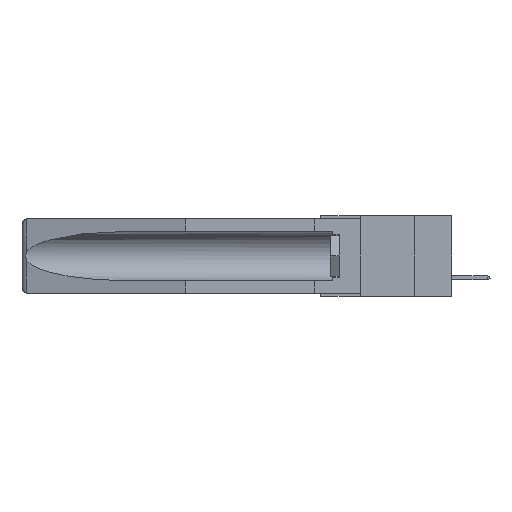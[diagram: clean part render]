
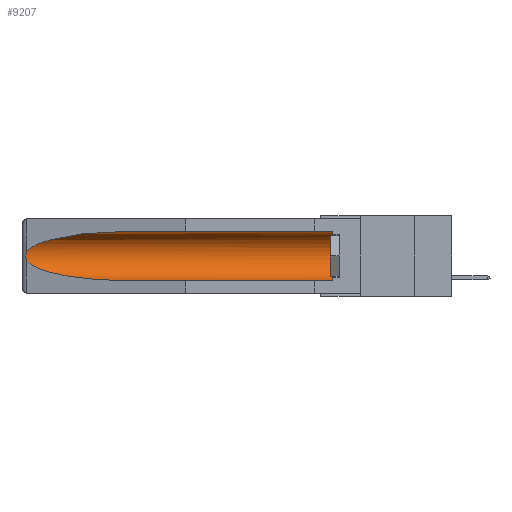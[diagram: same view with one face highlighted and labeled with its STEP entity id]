
A CAD part, left-side view. The second image highlights one B-rep face of the part: STEP entity #9207.
In plain terms, the highlighted cylindrical face has radius 2.857 mm (diameter 5.715 mm), a partial arc.
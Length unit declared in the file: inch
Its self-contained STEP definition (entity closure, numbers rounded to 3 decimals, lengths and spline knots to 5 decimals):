
#375 = B_SPLINE_CURVE_WITH_KNOTS ( 'NONE', 3,
 ( #19235, #2201, #18128, #20437, #11362, #25217, #8848, #13440, #29422, #16151 ),
 .UNSPECIFIED., .F., .F.,
 ( 4, 2, 2, 2, 4 ),
 ( 0., 0.00029, 0.00058, 0.00087, 0.00117 ),
 .UNSPECIFIED. ) ;
#1350 = ORIENTED_EDGE ( 'NONE', *, *, #18300, .T. ) ;
#1431 = VERTEX_POINT ( 'NONE', #3185 ) ;
#2054 = EDGE_CURVE ( 'NONE', #2586, #7337, #375, .T. ) ;
#2201 = CARTESIAN_POINT ( 'NONE',  ( 0.26597, 1.52961, -0.15275 ) ) ;
#2586 = VERTEX_POINT ( 'NONE', #4891 ) ;
#2819 = CARTESIAN_POINT ( 'NONE',  ( 0.155, 1.07973, -0.284 ) ) ;
#3185 = CARTESIAN_POINT ( 'NONE',  ( 0.155, 1.07973, -0.059 ) ) ;
#4318 = CARTESIAN_POINT ( 'NONE',  ( 0.155, 0.126, -0.059 ) ) ;
#4891 = CARTESIAN_POINT ( 'NONE',  ( 0.26537, 1.52718, -0.14972 ) ) ;
#6897 = CARTESIAN_POINT ( 'NONE',  ( 0.155, 0.126, -0.284 ) ) ;
#6979 =( BOUNDED_CURVE ( )  B_SPLINE_CURVE ( 3, ( #18238, #9272, #11580, #7093 ),
 .UNSPECIFIED., .F., .F. ) 
 B_SPLINE_CURVE_WITH_KNOTS ( ( 4, 4 ),
 ( 4.71239, 6.08839 ),
 .UNSPECIFIED. ) 
 CURVE ( )  GEOMETRIC_REPRESENTATION_ITEM ( )  RATIONAL_B_SPLINE_CURVE ( ( 1., 0.848, 0.848, 1. ) ) 
 REPRESENTATION_ITEM ( '' )  );
#7093 = CARTESIAN_POINT ( 'NONE',  ( 0.26537, 1.52718, -0.14972 ) ) ;
#7301 = CARTESIAN_POINT ( 'NONE',  ( 0.25451, 1.48313, -0.24835 ) ) ;
#7337 = VERTEX_POINT ( 'NONE', #17498 ) ;
#7455 = DIRECTION ( 'NONE',  ( 0., 1., 0. ) ) ;
#8050 = ORIENTED_EDGE ( 'NONE', *, *, #2054, .T. ) ;
#8314 = DIRECTION ( 'NONE',  ( 0., 1., 0. ) ) ;
#8575 = CARTESIAN_POINT ( 'NONE',  ( 0.155, 0.126, -0.1715 ) ) ;
#8848 = CARTESIAN_POINT ( 'NONE',  ( 0.2673, 1.53269, -0.17917 ) ) ;
#9207 = ADVANCED_FACE ( 'NONE', ( #29160 ), #17739, .F. ) ;
#9272 = CARTESIAN_POINT ( 'NONE',  ( 0.21114, 1.30732, -0.059 ) ) ;
#9380 = CARTESIAN_POINT ( 'NONE',  ( 0.26537, 1.52718, -0.19328 ) ) ;
#10042 = EDGE_CURVE ( 'NONE', #1431, #2586, #6979, .T. ) ;
#10326 = CARTESIAN_POINT ( 'NONE',  ( 0.155, -0.30754, -0.059 ) ) ;
#10507 = CARTESIAN_POINT ( 'NONE',  ( 0.155, -0.30754, -0.1715 ) ) ;
#11042 = ORIENTED_EDGE ( 'NONE', *, *, #27940, .F. ) ;
#11103 = EDGE_CURVE ( 'NONE', #11293, #22276, #15835, .T. ) ;
#11293 = VERTEX_POINT ( 'NONE', #6897 ) ;
#11362 = CARTESIAN_POINT ( 'NONE',  ( 0.2675, 1.53308, -0.16763 ) ) ;
#11580 = CARTESIAN_POINT ( 'NONE',  ( 0.25451, 1.48313, -0.09465 ) ) ;
#11657 = EDGE_CURVE ( 'NONE', #22276, #1431, #22636, .T. ) ;
#13177 = AXIS2_PLACEMENT_3D ( 'NONE', #10507, #17373, #26473 ) ;
#13263 = DIRECTION ( 'NONE',  ( 0., 0., 1. ) ) ;
#13440 = CARTESIAN_POINT ( 'NONE',  ( 0.26655, 1.53094, -0.18657 ) ) ;
#14767 = VECTOR ( 'NONE', #7455, 39.37008 ) ;
#15835 = CIRCLE ( 'NONE', #18563, 0.1125 ) ;
#16151 = CARTESIAN_POINT ( 'NONE',  ( 0.26537, 1.52718, -0.19328 ) ) ;
#17373 = DIRECTION ( 'NONE',  ( 0., 1., 0. ) ) ;
#17498 = CARTESIAN_POINT ( 'NONE',  ( 0.26537, 1.52718, -0.19328 ) ) ;
#17736 =( BOUNDED_CURVE ( )  B_SPLINE_CURVE ( 3, ( #9380, #7301, #18452, #18345 ),
 .UNSPECIFIED., .F., .F. ) 
 B_SPLINE_CURVE_WITH_KNOTS ( ( 4, 4 ),
 ( 0.1948, 1.5708 ),
 .UNSPECIFIED. ) 
 CURVE ( )  GEOMETRIC_REPRESENTATION_ITEM ( )  RATIONAL_B_SPLINE_CURVE ( ( 1., 0.848, 0.848, 1. ) ) 
 REPRESENTATION_ITEM ( '' )  );
#17739 = CYLINDRICAL_SURFACE ( 'NONE', #13177, 0.1125 ) ;
#18128 = CARTESIAN_POINT ( 'NONE',  ( 0.26654, 1.53092, -0.15636 ) ) ;
#18238 = CARTESIAN_POINT ( 'NONE',  ( 0.155, 1.07973, -0.059 ) ) ;
#18300 = EDGE_CURVE ( 'NONE', #7337, #28100, #17736, .T. ) ;
#18345 = CARTESIAN_POINT ( 'NONE',  ( 0.155, 1.07973, -0.284 ) ) ;
#18419 = CARTESIAN_POINT ( 'NONE',  ( 0.155, -0.30754, -0.284 ) ) ;
#18452 = CARTESIAN_POINT ( 'NONE',  ( 0.21114, 1.30732, -0.284 ) ) ;
#18563 = AXIS2_PLACEMENT_3D ( 'NONE', #8575, #24538, #13263 ) ;
#18629 = EDGE_LOOP ( 'NONE', ( #19105, #8050, #1350, #11042, #24296, #24566 ) ) ;
#19105 = ORIENTED_EDGE ( 'NONE', *, *, #10042, .T. ) ;
#19235 = CARTESIAN_POINT ( 'NONE',  ( 0.26537, 1.52718, -0.14972 ) ) ;
#20437 = CARTESIAN_POINT ( 'NONE',  ( 0.2673, 1.5327, -0.16383 ) ) ;
#20851 = LINE ( 'NONE', #18419, #14767 ) ;
#22276 = VERTEX_POINT ( 'NONE', #4318 ) ;
#22636 = LINE ( 'NONE', #10326, #25452 ) ;
#24296 = ORIENTED_EDGE ( 'NONE', *, *, #11103, .T. ) ;
#24538 = DIRECTION ( 'NONE',  ( 0., -1., 0. ) ) ;
#24566 = ORIENTED_EDGE ( 'NONE', *, *, #11657, .T. ) ;
#25217 = CARTESIAN_POINT ( 'NONE',  ( 0.2675, 1.53308, -0.17534 ) ) ;
#25452 = VECTOR ( 'NONE', #8314, 39.37008 ) ;
#26473 = DIRECTION ( 'NONE',  ( 0., 0., 1. ) ) ;
#27940 = EDGE_CURVE ( 'NONE', #11293, #28100, #20851, .T. ) ;
#28100 = VERTEX_POINT ( 'NONE', #2819 ) ;
#29160 = FACE_OUTER_BOUND ( 'NONE', #18629, .T. ) ;
#29422 = CARTESIAN_POINT ( 'NONE',  ( 0.26597, 1.5296, -0.19026 ) ) ;
